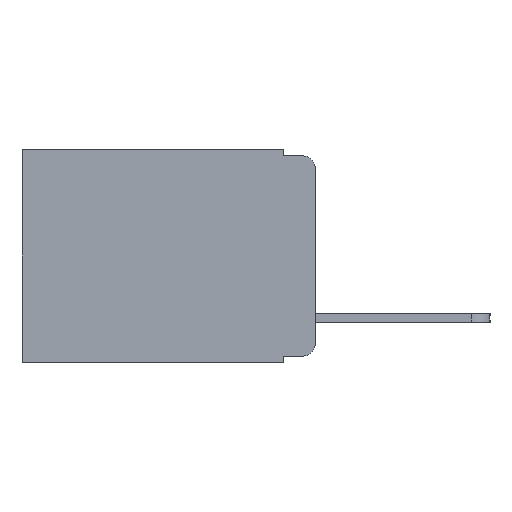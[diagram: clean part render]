
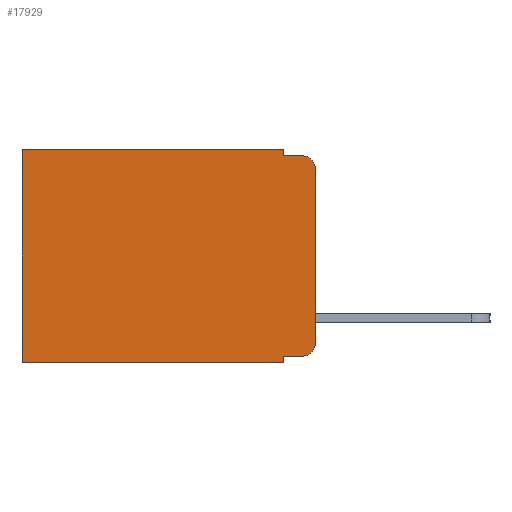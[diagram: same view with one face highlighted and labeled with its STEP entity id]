
A CAD part, left-side view. The second image highlights one B-rep face of the part: STEP entity #17929.
In plain terms, the highlighted planar face has unit normal (-1, 0, 0).
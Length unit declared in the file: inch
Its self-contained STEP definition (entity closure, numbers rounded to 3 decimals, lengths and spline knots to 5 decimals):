
#32 = ORIENTED_EDGE ( 'NONE', *, *, #8155, .T. ) ;
#189 = VECTOR ( 'NONE', #16246, 39.37008 ) ;
#366 = VERTEX_POINT ( 'NONE', #11727 ) ;
#868 = AXIS2_PLACEMENT_3D ( 'NONE', #16532, #15667, #5090 ) ;
#1275 = LINE ( 'NONE', #11525, #4980 ) ;
#1309 = VERTEX_POINT ( 'NONE', #14657 ) ;
#1484 = ORIENTED_EDGE ( 'NONE', *, *, #8077, .F. ) ;
#1531 = VERTEX_POINT ( 'NONE', #17279 ) ;
#1637 = DIRECTION ( 'NONE',  ( 0., 1., 0. ) ) ;
#2335 = VERTEX_POINT ( 'NONE', #6777 ) ;
#2389 = VERTEX_POINT ( 'NONE', #12339 ) ;
#2823 = CARTESIAN_POINT ( 'NONE',  ( 0.298, 0.473, 0. ) ) ;
#2939 = CARTESIAN_POINT ( 'NONE',  ( 0.298, 0., 0. ) ) ;
#3318 = CARTESIAN_POINT ( 'NONE',  ( 0.298, 0.02, -0.313 ) ) ;
#3581 = VECTOR ( 'NONE', #17439, 39.37008 ) ;
#3842 = PLANE ( 'NONE',  #7972 ) ;
#3938 = VERTEX_POINT ( 'NONE', #12640 ) ;
#4483 = LINE ( 'NONE', #2823, #11223 ) ;
#4980 = VECTOR ( 'NONE', #14101, 39.37008 ) ;
#5090 = DIRECTION ( 'NONE',  ( 0., 0., -1. ) ) ;
#5175 = ORIENTED_EDGE ( 'NONE', *, *, #7241, .T. ) ;
#5531 = VERTEX_POINT ( 'NONE', #15071 ) ;
#5563 = ORIENTED_EDGE ( 'NONE', *, *, #7755, .F. ) ;
#5871 = CARTESIAN_POINT ( 'NONE',  ( 0.298, 0.051, -0.01 ) ) ;
#6018 = VERTEX_POINT ( 'NONE', #15541 ) ;
#6752 = ORIENTED_EDGE ( 'NONE', *, *, #8026, .F. ) ;
#6761 = DIRECTION ( 'NONE',  ( 0., 0., -1. ) ) ;
#6777 = CARTESIAN_POINT ( 'NONE',  ( 0.298, 0.051, -0.333 ) ) ;
#7241 = EDGE_CURVE ( 'NONE', #6018, #2389, #10306, .T. ) ;
#7668 = VERTEX_POINT ( 'NONE', #16488 ) ;
#7755 = EDGE_CURVE ( 'NONE', #5531, #1309, #8706, .T. ) ;
#7972 = AXIS2_PLACEMENT_3D ( 'NONE', #17094, #14480, #6761 ) ;
#8026 = EDGE_CURVE ( 'NONE', #3938, #1531, #13281, .T. ) ;
#8052 = EDGE_CURVE ( 'NONE', #3938, #7668, #9516, .T. ) ;
#8077 = EDGE_CURVE ( 'NONE', #12322, #7668, #1275, .T. ) ;
#8103 = EDGE_CURVE ( 'NONE', #6018, #12322, #11637, .T. ) ;
#8106 = EDGE_CURVE ( 'NONE', #2389, #1309, #4483, .T. ) ;
#8129 = EDGE_CURVE ( 'NONE', #2335, #5531, #14649, .T. ) ;
#8135 = EDGE_CURVE ( 'NONE', #2335, #366, #10852, .T. ) ;
#8155 = EDGE_CURVE ( 'NONE', #366, #1531, #13840, .T. ) ;
#8536 = ORIENTED_EDGE ( 'NONE', *, *, #8103, .F. ) ;
#8706 = LINE ( 'NONE', #10265, #15508 ) ;
#9501 = ORIENTED_EDGE ( 'NONE', *, *, #8135, .T. ) ;
#9516 = CIRCLE ( 'NONE', #868, 0.02 ) ;
#9678 = AXIS2_PLACEMENT_3D ( 'NONE', #3318, #15487, #15401 ) ;
#9797 = DIRECTION ( 'NONE',  ( 0., 0., -1. ) ) ;
#9851 = CARTESIAN_POINT ( 'NONE',  ( 0.298, 0.051, 0. ) ) ;
#10265 = CARTESIAN_POINT ( 'NONE',  ( 0.298, 0., -0.343 ) ) ;
#10286 = DIRECTION ( 'NONE',  ( 0., 1., 0. ) ) ;
#10306 = LINE ( 'NONE', #2939, #16767 ) ;
#10852 = LINE ( 'NONE', #17420, #3581 ) ;
#11088 = ORIENTED_EDGE ( 'NONE', *, *, #8052, .T. ) ;
#11124 = ORIENTED_EDGE ( 'NONE', *, *, #8129, .F. ) ;
#11223 = VECTOR ( 'NONE', #9797, 39.37008 ) ;
#11525 = CARTESIAN_POINT ( 'NONE',  ( 0.298, 0.051, -0.01 ) ) ;
#11637 = LINE ( 'NONE', #13948, #189 ) ;
#11727 = CARTESIAN_POINT ( 'NONE',  ( 0.298, 0.02, -0.333 ) ) ;
#11961 = DIRECTION ( 'NONE',  ( 0., 0., -1. ) ) ;
#12322 = VERTEX_POINT ( 'NONE', #5871 ) ;
#12339 = CARTESIAN_POINT ( 'NONE',  ( 0.298, 0.473, 0. ) ) ;
#12640 = CARTESIAN_POINT ( 'NONE',  ( 0.298, 0., -0.03 ) ) ;
#13281 = LINE ( 'NONE', #14483, #15888 ) ;
#13472 = ORIENTED_EDGE ( 'NONE', *, *, #8106, .T. ) ;
#13840 = CIRCLE ( 'NONE', #9678, 0.02 ) ;
#13948 = CARTESIAN_POINT ( 'NONE',  ( 0.298, 0.051, 0. ) ) ;
#14101 = DIRECTION ( 'NONE',  ( 0., -1., 0. ) ) ;
#14228 = VECTOR ( 'NONE', #15831, 39.37008 ) ;
#14480 = DIRECTION ( 'NONE',  ( 1., 0., 0. ) ) ;
#14483 = CARTESIAN_POINT ( 'NONE',  ( 0.298, 0., 0. ) ) ;
#14649 = LINE ( 'NONE', #9851, #14228 ) ;
#14657 = CARTESIAN_POINT ( 'NONE',  ( 0.298, 0.473, -0.343 ) ) ;
#15071 = CARTESIAN_POINT ( 'NONE',  ( 0.298, 0.051, -0.343 ) ) ;
#15401 = DIRECTION ( 'NONE',  ( 0., 0., -1. ) ) ;
#15487 = DIRECTION ( 'NONE',  ( -1., 0., 0. ) ) ;
#15508 = VECTOR ( 'NONE', #10286, 39.37008 ) ;
#15541 = CARTESIAN_POINT ( 'NONE',  ( 0.298, 0.051, 0. ) ) ;
#15667 = DIRECTION ( 'NONE',  ( -1., 0., 0. ) ) ;
#15831 = DIRECTION ( 'NONE',  ( 0., 0., -1. ) ) ;
#15888 = VECTOR ( 'NONE', #11961, 39.37008 ) ;
#16246 = DIRECTION ( 'NONE',  ( 0., 0., -1. ) ) ;
#16382 = FACE_OUTER_BOUND ( 'NONE', #16582, .T. ) ;
#16488 = CARTESIAN_POINT ( 'NONE',  ( 0.298, 0.02, -0.01 ) ) ;
#16532 = CARTESIAN_POINT ( 'NONE',  ( 0.298, 0.02, -0.03 ) ) ;
#16582 = EDGE_LOOP ( 'NONE', ( #6752, #11088, #1484, #8536, #5175, #13472, #5563, #11124, #9501, #32 ) ) ;
#16767 = VECTOR ( 'NONE', #1637, 39.37008 ) ;
#17094 = CARTESIAN_POINT ( 'NONE',  ( 0.298, 0., 0. ) ) ;
#17279 = CARTESIAN_POINT ( 'NONE',  ( 0.298, 0., -0.313 ) ) ;
#17420 = CARTESIAN_POINT ( 'NONE',  ( 0.298, 0.051, -0.333 ) ) ;
#17439 = DIRECTION ( 'NONE',  ( 0., -1., 0. ) ) ;
#17929 = ADVANCED_FACE ( 'NONE', ( #16382 ), #3842, .F. ) ;
